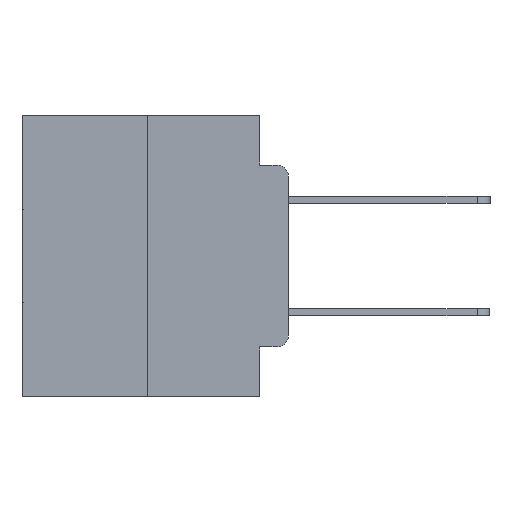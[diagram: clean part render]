
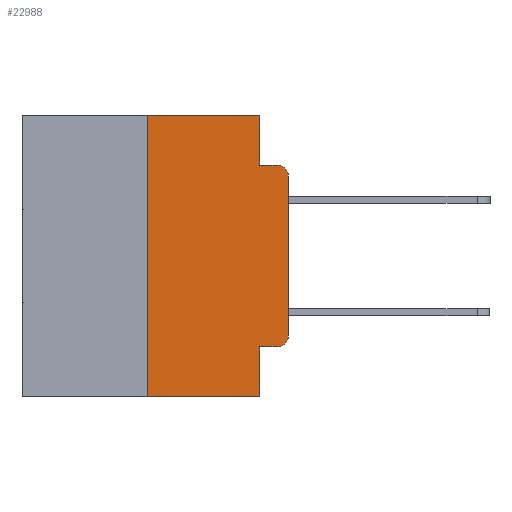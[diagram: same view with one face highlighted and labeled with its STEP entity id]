
A CAD part, left-side view. The second image highlights one B-rep face of the part: STEP entity #22988.
In plain terms, the highlighted planar face has unit normal (-1, 0, 0).
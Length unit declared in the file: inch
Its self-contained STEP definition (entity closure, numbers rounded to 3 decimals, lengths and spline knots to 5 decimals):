
#42 = EDGE_CURVE ( 'NONE', #15935, #8558, #11273, .T. ) ;
#471 = ORIENTED_EDGE ( 'NONE', *, *, #9715, .T. ) ;
#1306 = VERTEX_POINT ( 'NONE', #5829 ) ;
#1609 = VERTEX_POINT ( 'NONE', #13489 ) ;
#2029 = LINE ( 'NONE', #9801, #24968 ) ;
#2497 = DIRECTION ( 'NONE',  ( 0., -1., 0. ) ) ;
#3241 = VERTEX_POINT ( 'NONE', #16927 ) ;
#3777 = AXIS2_PLACEMENT_3D ( 'NONE', #21220, #8088, #23397 ) ;
#4424 = CARTESIAN_POINT ( 'NONE',  ( 0., 0.473, 0. ) ) ;
#4598 = CIRCLE ( 'NONE', #3777, 0.02 ) ;
#4831 = LINE ( 'NONE', #4424, #21093 ) ;
#5389 = CARTESIAN_POINT ( 'NONE',  ( 0., 0., 0. ) ) ;
#5390 = VERTEX_POINT ( 'NONE', #25306 ) ;
#5565 = ORIENTED_EDGE ( 'NONE', *, *, #9462, .F. ) ;
#5804 = EDGE_CURVE ( 'NONE', #15928, #1609, #10998, .T. ) ;
#5829 = CARTESIAN_POINT ( 'NONE',  ( 0., 0.02, -0.4115 ) ) ;
#5979 = VERTEX_POINT ( 'NONE', #18636 ) ;
#6068 = CARTESIAN_POINT ( 'NONE',  ( 0., 0.473, -0.5 ) ) ;
#6117 = CARTESIAN_POINT ( 'NONE',  ( 0., 0.25, 0. ) ) ;
#6685 = CARTESIAN_POINT ( 'NONE',  ( 0., 0.473, 0. ) ) ;
#7066 = CARTESIAN_POINT ( 'NONE',  ( 0., 0.25, -0.5 ) ) ;
#8088 = DIRECTION ( 'NONE',  ( -1., 0., 0. ) ) ;
#8558 = VERTEX_POINT ( 'NONE', #28136 ) ;
#9019 = DIRECTION ( 'NONE',  ( 0., 0., -1. ) ) ;
#9295 = CARTESIAN_POINT ( 'NONE',  ( 0., 0.02, -0.1085 ) ) ;
#9336 = LINE ( 'NONE', #22819, #14481 ) ;
#9462 = EDGE_CURVE ( 'NONE', #5979, #3241, #2029, .T. ) ;
#9627 = EDGE_CURVE ( 'NONE', #1306, #5390, #4598, .T. ) ;
#9715 = EDGE_CURVE ( 'NONE', #15935, #28778, #18844, .T. ) ;
#9801 = CARTESIAN_POINT ( 'NONE',  ( 0., 0.051, 0. ) ) ;
#10219 = CARTESIAN_POINT ( 'NONE',  ( 0., 0.051, -0.4115 ) ) ;
#10998 = CIRCLE ( 'NONE', #12684, 0.02 ) ;
#11273 = LINE ( 'NONE', #6117, #21442 ) ;
#11446 = AXIS2_PLACEMENT_3D ( 'NONE', #6685, #22096, #9019 ) ;
#11534 = DIRECTION ( 'NONE',  ( 0., 0., -1. ) ) ;
#11649 = CARTESIAN_POINT ( 'NONE',  ( 0., 0., -0.1085 ) ) ;
#11731 = EDGE_CURVE ( 'NONE', #5390, #15928, #18386, .T. ) ;
#11938 = DIRECTION ( 'NONE',  ( 0., -1., 0. ) ) ;
#12035 = DIRECTION ( 'NONE',  ( 0., 0., -1. ) ) ;
#12633 = VECTOR ( 'NONE', #16585, 39.37008 ) ;
#12684 = AXIS2_PLACEMENT_3D ( 'NONE', #9295, #24527, #11534 ) ;
#12966 = CARTESIAN_POINT ( 'NONE',  ( 0., 0.051, -0.5 ) ) ;
#13489 = CARTESIAN_POINT ( 'NONE',  ( 0., 0.02, -0.0885 ) ) ;
#13763 = VECTOR ( 'NONE', #23582, 39.37008 ) ;
#14481 = VECTOR ( 'NONE', #11938, 39.37008 ) ;
#15549 = EDGE_CURVE ( 'NONE', #8558, #5979, #4831, .T. ) ;
#15928 = VERTEX_POINT ( 'NONE', #11649 ) ;
#15935 = VERTEX_POINT ( 'NONE', #7066 ) ;
#16001 = CARTESIAN_POINT ( 'NONE',  ( 0., 0.051, -0.4115 ) ) ;
#16100 = ORIENTED_EDGE ( 'NONE', *, *, #42, .F. ) ;
#16414 = EDGE_CURVE ( 'NONE', #27096, #1306, #22411, .T. ) ;
#16559 = VECTOR ( 'NONE', #24669, 39.37008 ) ;
#16585 = DIRECTION ( 'NONE',  ( 0., 0., 1. ) ) ;
#16642 = VECTOR ( 'NONE', #2497, 39.37008 ) ;
#16927 = CARTESIAN_POINT ( 'NONE',  ( 0., 0.051, -0.0885 ) ) ;
#17492 = FACE_OUTER_BOUND ( 'NONE', #17952, .T. ) ;
#17952 = EDGE_LOOP ( 'NONE', ( #22018, #23716, #27514, #5565, #21129, #16100, #471, #25733, #28675, #22233 ) ) ;
#18386 = LINE ( 'NONE', #5389, #12633 ) ;
#18636 = CARTESIAN_POINT ( 'NONE',  ( 0., 0.051, 0. ) ) ;
#18844 = LINE ( 'NONE', #6068, #13763 ) ;
#20754 = EDGE_CURVE ( 'NONE', #27096, #28778, #21642, .T. ) ;
#21093 = VECTOR ( 'NONE', #22138, 39.37008 ) ;
#21129 = ORIENTED_EDGE ( 'NONE', *, *, #15549, .F. ) ;
#21220 = CARTESIAN_POINT ( 'NONE',  ( 0., 0.02, -0.3915 ) ) ;
#21442 = VECTOR ( 'NONE', #28416, 39.37008 ) ;
#21642 = LINE ( 'NONE', #24570, #16559 ) ;
#22007 = PLANE ( 'NONE',  #11446 ) ;
#22018 = ORIENTED_EDGE ( 'NONE', *, *, #11731, .T. ) ;
#22096 = DIRECTION ( 'NONE',  ( 1., 0., 0. ) ) ;
#22138 = DIRECTION ( 'NONE',  ( 0., -1., 0. ) ) ;
#22233 = ORIENTED_EDGE ( 'NONE', *, *, #9627, .T. ) ;
#22411 = LINE ( 'NONE', #16001, #16642 ) ;
#22819 = CARTESIAN_POINT ( 'NONE',  ( 0., 0.051, -0.0885 ) ) ;
#22988 = ADVANCED_FACE ( 'NONE', ( #17492 ), #22007, .F. ) ;
#23397 = DIRECTION ( 'NONE',  ( 0., 0., -1. ) ) ;
#23582 = DIRECTION ( 'NONE',  ( 0., -1., 0. ) ) ;
#23716 = ORIENTED_EDGE ( 'NONE', *, *, #5804, .T. ) ;
#24527 = DIRECTION ( 'NONE',  ( -1., 0., 0. ) ) ;
#24570 = CARTESIAN_POINT ( 'NONE',  ( 0., 0.051, 0. ) ) ;
#24669 = DIRECTION ( 'NONE',  ( 0., 0., -1. ) ) ;
#24968 = VECTOR ( 'NONE', #12035, 39.37008 ) ;
#25306 = CARTESIAN_POINT ( 'NONE',  ( 0., 0., -0.3915 ) ) ;
#25733 = ORIENTED_EDGE ( 'NONE', *, *, #20754, .F. ) ;
#27096 = VERTEX_POINT ( 'NONE', #10219 ) ;
#27514 = ORIENTED_EDGE ( 'NONE', *, *, #28466, .F. ) ;
#28136 = CARTESIAN_POINT ( 'NONE',  ( 0., 0.25, 0. ) ) ;
#28416 = DIRECTION ( 'NONE',  ( 0., 0., 1. ) ) ;
#28466 = EDGE_CURVE ( 'NONE', #3241, #1609, #9336, .T. ) ;
#28675 = ORIENTED_EDGE ( 'NONE', *, *, #16414, .T. ) ;
#28778 = VERTEX_POINT ( 'NONE', #12966 ) ;
